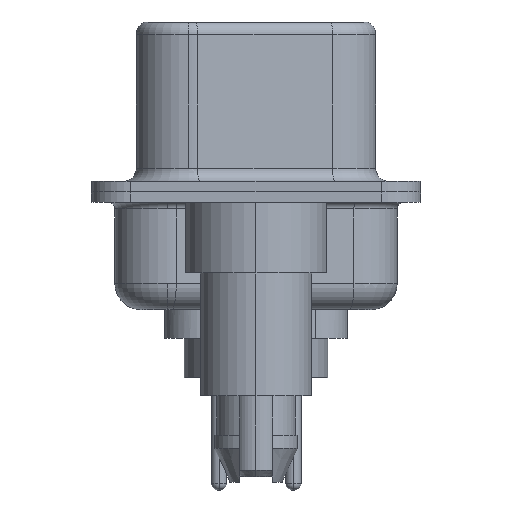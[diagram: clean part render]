
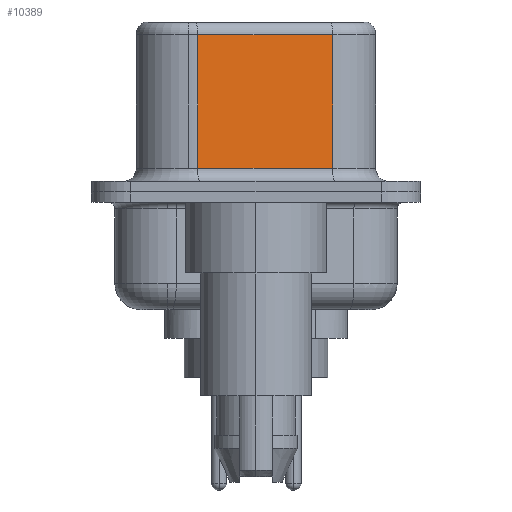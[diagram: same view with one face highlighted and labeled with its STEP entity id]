
A CAD part, left-side view. The second image highlights one B-rep face of the part: STEP entity #10389.
In plain terms, the highlighted planar face has unit normal (-0.985, -0.174, 0).
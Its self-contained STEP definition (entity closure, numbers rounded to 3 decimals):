
#1400 = CARTESIAN_POINT ( 'NONE',  ( 4.565, -2.927, 6.02 ) ) ;
#2324 = EDGE_LOOP ( 'NONE', ( #8762, #19944, #5298, #2809 ) ) ;
#2589 = VERTEX_POINT ( 'NONE', #4482 ) ;
#2672 = DIRECTION ( 'NONE',  ( 0., 0., -1. ) ) ;
#2687 = CARTESIAN_POINT ( 'NONE',  ( 4.565, -2.927, 0.9 ) ) ;
#2809 = ORIENTED_EDGE ( 'NONE', *, *, #4326, .T. ) ;
#2972 = DIRECTION ( 'NONE',  ( -0.174, 0.985, 0. ) ) ;
#4326 = EDGE_CURVE ( 'NONE', #2589, #7403, #5700, .T. ) ;
#4482 = CARTESIAN_POINT ( 'NONE',  ( 3.655, 2.233, 0.9 ) ) ;
#4859 = VECTOR ( 'NONE', #2672, 1000. ) ;
#5069 = EDGE_CURVE ( 'NONE', #15808, #8106, #8422, .T. ) ;
#5298 = ORIENTED_EDGE ( 'NONE', *, *, #10113, .T. ) ;
#5700 = LINE ( 'NONE', #15774, #17874 ) ;
#6142 = CARTESIAN_POINT ( 'NONE',  ( 4.565, -2.927, 6.52 ) ) ;
#6514 = AXIS2_PLACEMENT_3D ( 'NONE', #6142, #12527, #2972 ) ;
#7403 = VERTEX_POINT ( 'NONE', #2687 ) ;
#7566 = EDGE_CURVE ( 'NONE', #15808, #7403, #13327, .T. ) ;
#7796 = FACE_OUTER_BOUND ( 'NONE', #2324, .T. ) ;
#8106 = VERTEX_POINT ( 'NONE', #18104 ) ;
#8422 = LINE ( 'NONE', #1400, #16860 ) ;
#8762 = ORIENTED_EDGE ( 'NONE', *, *, #7566, .F. ) ;
#9053 = CARTESIAN_POINT ( 'NONE',  ( 4.565, -2.927, 6.52 ) ) ;
#10113 = EDGE_CURVE ( 'NONE', #8106, #2589, #19778, .T. ) ;
#10389 = ADVANCED_FACE ( 'NONE', ( #7796 ), #10958, .F. ) ;
#10958 = PLANE ( 'NONE',  #6514 ) ;
#11770 = VECTOR ( 'NONE', #15022, 1000. ) ;
#12527 = DIRECTION ( 'NONE',  ( 0.985, 0.174, 0. ) ) ;
#13327 = LINE ( 'NONE', #9053, #4859 ) ;
#14102 = DIRECTION ( 'NONE',  ( -0.174, 0.985, 0. ) ) ;
#14843 = DIRECTION ( 'NONE',  ( 0.174, -0.985, 0. ) ) ;
#15022 = DIRECTION ( 'NONE',  ( 0., 0., -1. ) ) ;
#15774 = CARTESIAN_POINT ( 'NONE',  ( 4.565, -2.927, 0.9 ) ) ;
#15808 = VERTEX_POINT ( 'NONE', #17307 ) ;
#16653 = CARTESIAN_POINT ( 'NONE',  ( 3.655, 2.233, 6.52 ) ) ;
#16860 = VECTOR ( 'NONE', #14102, 1000. ) ;
#17307 = CARTESIAN_POINT ( 'NONE',  ( 4.565, -2.927, 6.02 ) ) ;
#17874 = VECTOR ( 'NONE', #14843, 1000. ) ;
#18104 = CARTESIAN_POINT ( 'NONE',  ( 3.655, 2.233, 6.02 ) ) ;
#19778 = LINE ( 'NONE', #16653, #11770 ) ;
#19944 = ORIENTED_EDGE ( 'NONE', *, *, #5069, .T. ) ;
